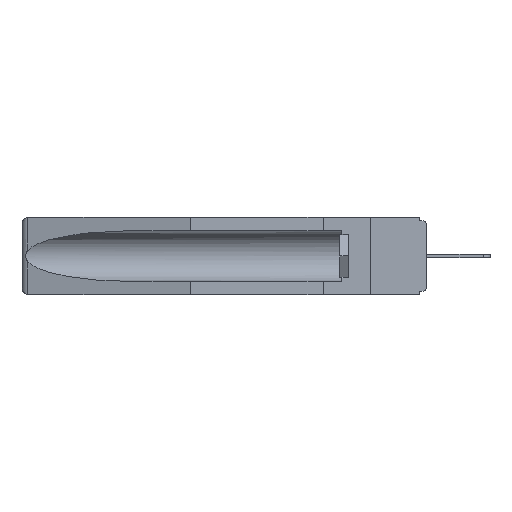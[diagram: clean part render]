
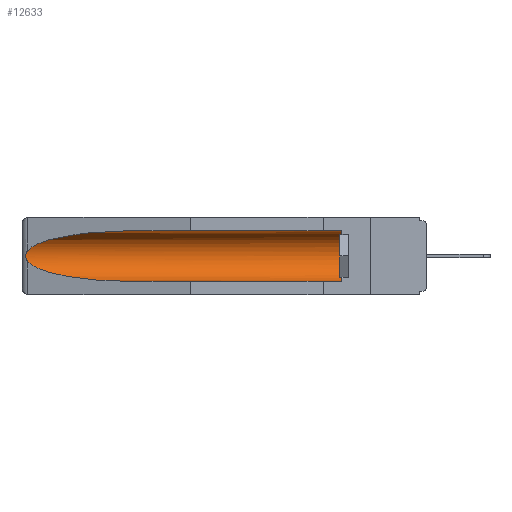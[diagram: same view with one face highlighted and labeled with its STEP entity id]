
A CAD part, left-side view. The second image highlights one B-rep face of the part: STEP entity #12633.
In plain terms, the highlighted cylindrical face has radius 2.857 mm (diameter 5.715 mm), a partial arc.
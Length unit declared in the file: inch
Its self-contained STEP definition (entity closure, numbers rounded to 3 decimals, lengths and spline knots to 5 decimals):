
#463 = VERTEX_POINT ( 'NONE', #8229 ) ;
#1479 = LINE ( 'NONE', #14306, #6442 ) ;
#1647 = CARTESIAN_POINT ( 'NONE',  ( 0.26537, 1.52718, -0.19328 ) ) ;
#1798 = LINE ( 'NONE', #17222, #12787 ) ;
#2193 = ORIENTED_EDGE ( 'NONE', *, *, #17337, .F. ) ;
#2434 = ORIENTED_EDGE ( 'NONE', *, *, #16887, .T. ) ;
#3157 = FACE_OUTER_BOUND ( 'NONE', #4841, .T. ) ;
#3198 = CARTESIAN_POINT ( 'NONE',  ( 0.26537, 1.52718, -0.14972 ) ) ;
#3752 = CARTESIAN_POINT ( 'NONE',  ( 0.155, 0.126, -0.1715 ) ) ;
#4186 = VERTEX_POINT ( 'NONE', #3198 ) ;
#4660 = VERTEX_POINT ( 'NONE', #4970 ) ;
#4841 = EDGE_LOOP ( 'NONE', ( #9863, #2434, #16622, #2193, #16744, #15602 ) ) ;
#4954 = CARTESIAN_POINT ( 'NONE',  ( 0.155, 0.126, -0.284 ) ) ;
#4970 = CARTESIAN_POINT ( 'NONE',  ( 0.26537, 1.52718, -0.19328 ) ) ;
#4971 = DIRECTION ( 'NONE',  ( 0., 1., 0. ) ) ;
#5242 = DIRECTION ( 'NONE',  ( 0., 0., 1. ) ) ;
#5331 = DIRECTION ( 'NONE',  ( 0., 1., 0. ) ) ;
#5529 = CARTESIAN_POINT ( 'NONE',  ( 0.25451, 1.48313, -0.09465 ) ) ;
#5622 = CARTESIAN_POINT ( 'NONE',  ( 0.2673, 1.5327, -0.16383 ) ) ;
#5866 = EDGE_CURVE ( 'NONE', #9593, #463, #1479, .T. ) ;
#6189 = CARTESIAN_POINT ( 'NONE',  ( 0.21114, 1.30732, -0.284 ) ) ;
#6380 = VERTEX_POINT ( 'NONE', #4954 ) ;
#6442 = VECTOR ( 'NONE', #15774, 39.37008 ) ;
#6842 = CARTESIAN_POINT ( 'NONE',  ( 0.155, 1.07973, -0.284 ) ) ;
#7044 = EDGE_CURVE ( 'NONE', #6380, #9593, #15931, .T. ) ;
#7148 = CARTESIAN_POINT ( 'NONE',  ( 0.2675, 1.53308, -0.17534 ) ) ;
#8015 = CARTESIAN_POINT ( 'NONE',  ( 0.155, -0.30754, -0.1715 ) ) ;
#8229 = CARTESIAN_POINT ( 'NONE',  ( 0.155, 1.07973, -0.059 ) ) ;
#8608 = CARTESIAN_POINT ( 'NONE',  ( 0.26537, 1.52718, -0.14972 ) ) ;
#8672 = CARTESIAN_POINT ( 'NONE',  ( 0.26655, 1.53094, -0.18657 ) ) ;
#8754 = EDGE_CURVE ( 'NONE', #463, #4186, #15192, .T. ) ;
#9593 = VERTEX_POINT ( 'NONE', #17813 ) ;
#9863 = ORIENTED_EDGE ( 'NONE', *, *, #8754, .T. ) ;
#10102 = AXIS2_PLACEMENT_3D ( 'NONE', #3752, #14193, #5242 ) ;
#10164 = CARTESIAN_POINT ( 'NONE',  ( 0.26537, 1.52718, -0.19328 ) ) ;
#11466 = CARTESIAN_POINT ( 'NONE',  ( 0.155, 1.07973, -0.059 ) ) ;
#12633 = ADVANCED_FACE ( 'NONE', ( #3157 ), #14605, .F. ) ;
#12787 = VECTOR ( 'NONE', #5331, 39.37008 ) ;
#13613 = CARTESIAN_POINT ( 'NONE',  ( 0.25451, 1.48313, -0.24835 ) ) ;
#13796 = EDGE_CURVE ( 'NONE', #4660, #16691, #14244, .T. ) ;
#14193 = DIRECTION ( 'NONE',  ( 0., -1., 0. ) ) ;
#14244 =( BOUNDED_CURVE ( )  B_SPLINE_CURVE ( 3, ( #1647, #13613, #6189, #16577 ),
 .UNSPECIFIED., .F., .F. ) 
 B_SPLINE_CURVE_WITH_KNOTS ( ( 4, 4 ),
 ( 0.1948, 1.5708 ),
 .UNSPECIFIED. ) 
 CURVE ( )  GEOMETRIC_REPRESENTATION_ITEM ( )  RATIONAL_B_SPLINE_CURVE ( ( 1., 0.848, 0.848, 1. ) ) 
 REPRESENTATION_ITEM ( '' )  );
#14306 = CARTESIAN_POINT ( 'NONE',  ( 0.155, -0.30754, -0.059 ) ) ;
#14471 = CARTESIAN_POINT ( 'NONE',  ( 0.21114, 1.30732, -0.059 ) ) ;
#14500 = CARTESIAN_POINT ( 'NONE',  ( 0.26597, 1.52961, -0.15275 ) ) ;
#14557 = CARTESIAN_POINT ( 'NONE',  ( 0.26654, 1.53092, -0.15636 ) ) ;
#14605 = CYLINDRICAL_SURFACE ( 'NONE', #14785, 0.1125 ) ;
#14785 = AXIS2_PLACEMENT_3D ( 'NONE', #8015, #4971, #18350 ) ;
#15192 =( BOUNDED_CURVE ( )  B_SPLINE_CURVE ( 3, ( #11466, #14471, #5529, #15938 ),
 .UNSPECIFIED., .F., .T. ) 
 B_SPLINE_CURVE_WITH_KNOTS ( ( 4, 4 ),
 ( 4.71239, 6.08839 ),
 .UNSPECIFIED. ) 
 CURVE ( )  GEOMETRIC_REPRESENTATION_ITEM ( )  RATIONAL_B_SPLINE_CURVE ( ( 1., 0.848, 0.848, 1. ) ) 
 REPRESENTATION_ITEM ( '' )  );
#15602 = ORIENTED_EDGE ( 'NONE', *, *, #5866, .T. ) ;
#15774 = DIRECTION ( 'NONE',  ( 0., 1., 0. ) ) ;
#15931 = CIRCLE ( 'NONE', #10102, 0.1125 ) ;
#15938 = CARTESIAN_POINT ( 'NONE',  ( 0.26537, 1.52718, -0.14972 ) ) ;
#16035 = CARTESIAN_POINT ( 'NONE',  ( 0.2675, 1.53308, -0.16763 ) ) ;
#16577 = CARTESIAN_POINT ( 'NONE',  ( 0.155, 1.07973, -0.284 ) ) ;
#16622 = ORIENTED_EDGE ( 'NONE', *, *, #13796, .T. ) ;
#16691 = VERTEX_POINT ( 'NONE', #6842 ) ;
#16716 = B_SPLINE_CURVE_WITH_KNOTS ( 'NONE', 3,
 ( #8608, #14500, #14557, #5622, #16035, #7148, #17487, #8672, #18991, #10164 ),
 .UNSPECIFIED., .F., .F.,
 ( 4, 2, 2, 2, 4 ),
 ( 0., 0.00029, 0.00058, 0.00087, 0.00117 ),
 .UNSPECIFIED. ) ;
#16744 = ORIENTED_EDGE ( 'NONE', *, *, #7044, .T. ) ;
#16887 = EDGE_CURVE ( 'NONE', #4186, #4660, #16716, .T. ) ;
#17222 = CARTESIAN_POINT ( 'NONE',  ( 0.155, -0.30754, -0.284 ) ) ;
#17337 = EDGE_CURVE ( 'NONE', #6380, #16691, #1798, .T. ) ;
#17487 = CARTESIAN_POINT ( 'NONE',  ( 0.2673, 1.53269, -0.17917 ) ) ;
#17813 = CARTESIAN_POINT ( 'NONE',  ( 0.155, 0.126, -0.059 ) ) ;
#18350 = DIRECTION ( 'NONE',  ( 0., 0., 1. ) ) ;
#18991 = CARTESIAN_POINT ( 'NONE',  ( 0.26597, 1.5296, -0.19026 ) ) ;
